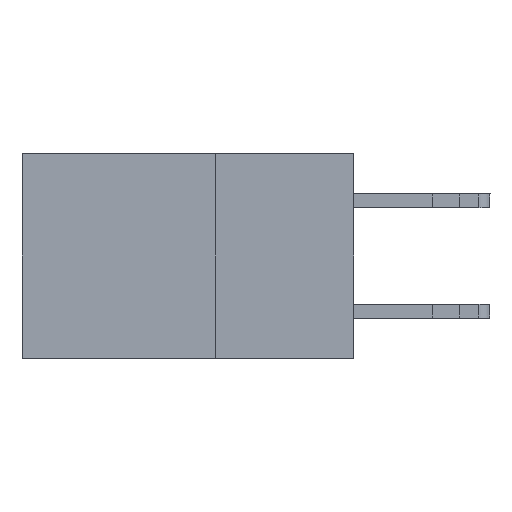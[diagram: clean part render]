
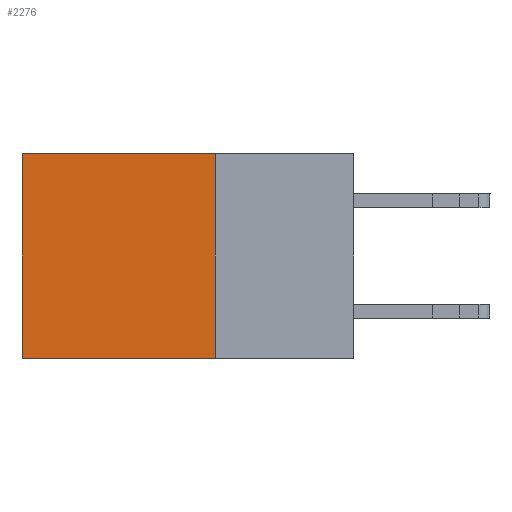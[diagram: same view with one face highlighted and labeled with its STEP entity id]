
A CAD part, left-side view. The second image highlights one B-rep face of the part: STEP entity #2276.
In plain terms, the highlighted planar face has unit normal (-1, 0, 0).
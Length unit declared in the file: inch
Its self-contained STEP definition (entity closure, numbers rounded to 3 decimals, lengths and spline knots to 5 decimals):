
#276 = CARTESIAN_POINT ( 'NONE',  ( 0.2875, 0.6, 0. ) ) ;
#328 = EDGE_CURVE ( 'NONE', #17053, #18104, #29896, .T. ) ;
#1016 = ORIENTED_EDGE ( 'NONE', *, *, #12004, .F. ) ;
#2276 = ADVANCED_FACE ( 'NONE', ( #16999 ), #9821, .F. ) ;
#3684 = EDGE_CURVE ( 'NONE', #9748, #18104, #5037, .T. ) ;
#3710 = ORIENTED_EDGE ( 'NONE', *, *, #21984, .T. ) ;
#4614 = EDGE_LOOP ( 'NONE', ( #13524, #9592, #1016, #3710 ) ) ;
#5037 = LINE ( 'NONE', #276, #9294 ) ;
#5427 = VECTOR ( 'NONE', #19382, 39.37008 ) ;
#6135 = LINE ( 'NONE', #12096, #20094 ) ;
#7519 = AXIS2_PLACEMENT_3D ( 'NONE', #7541, #20045, #16421 ) ;
#7541 = CARTESIAN_POINT ( 'NONE',  ( 0.2875, 0.25, 0. ) ) ;
#7814 = CARTESIAN_POINT ( 'NONE',  ( 0.2875, 0.25, 0. ) ) ;
#9294 = VECTOR ( 'NONE', #25136, 39.37008 ) ;
#9358 = CARTESIAN_POINT ( 'NONE',  ( 0.2875, 0.25, 0. ) ) ;
#9592 = ORIENTED_EDGE ( 'NONE', *, *, #328, .F. ) ;
#9748 = VERTEX_POINT ( 'NONE', #23078 ) ;
#9821 = PLANE ( 'NONE',  #7519 ) ;
#12004 = EDGE_CURVE ( 'NONE', #14673, #17053, #18624, .T. ) ;
#12096 = CARTESIAN_POINT ( 'NONE',  ( 0.2875, 0.25, 0. ) ) ;
#13524 = ORIENTED_EDGE ( 'NONE', *, *, #3684, .T. ) ;
#14673 = VERTEX_POINT ( 'NONE', #7814 ) ;
#16421 = DIRECTION ( 'NONE',  ( 0., 0., -1. ) ) ;
#16999 = FACE_OUTER_BOUND ( 'NONE', #4614, .T. ) ;
#17053 = VERTEX_POINT ( 'NONE', #28361 ) ;
#18104 = VERTEX_POINT ( 'NONE', #27828 ) ;
#18624 = LINE ( 'NONE', #9358, #5427 ) ;
#19382 = DIRECTION ( 'NONE',  ( 0., 0., -1. ) ) ;
#20045 = DIRECTION ( 'NONE',  ( 1., 0., 0. ) ) ;
#20094 = VECTOR ( 'NONE', #31875, 39.37008 ) ;
#21984 = EDGE_CURVE ( 'NONE', #14673, #9748, #6135, .T. ) ;
#22338 = CARTESIAN_POINT ( 'NONE',  ( 0.2875, 0.25, -0.37 ) ) ;
#22663 = DIRECTION ( 'NONE',  ( 0., 1., 0. ) ) ;
#23078 = CARTESIAN_POINT ( 'NONE',  ( 0.2875, 0.6, 0. ) ) ;
#25136 = DIRECTION ( 'NONE',  ( 0., 0., -1. ) ) ;
#25633 = VECTOR ( 'NONE', #22663, 39.37008 ) ;
#27828 = CARTESIAN_POINT ( 'NONE',  ( 0.2875, 0.6, -0.37 ) ) ;
#28361 = CARTESIAN_POINT ( 'NONE',  ( 0.2875, 0.25, -0.37 ) ) ;
#29896 = LINE ( 'NONE', #22338, #25633 ) ;
#31875 = DIRECTION ( 'NONE',  ( 0., 1., 0. ) ) ;
